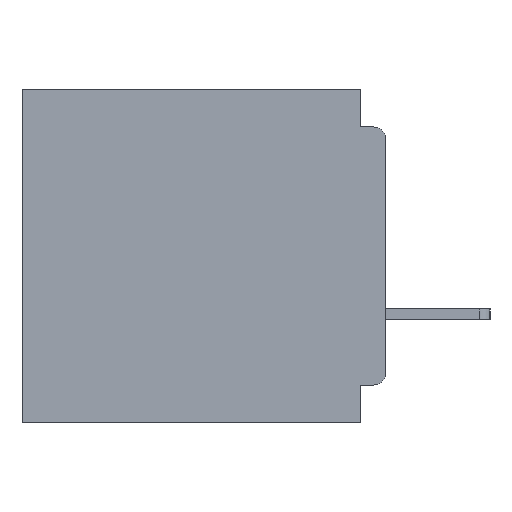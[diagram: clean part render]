
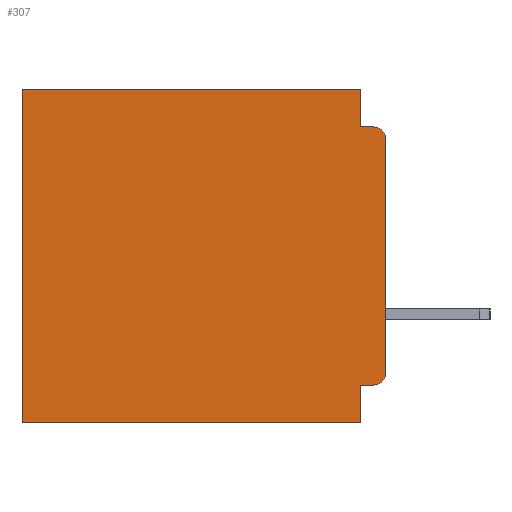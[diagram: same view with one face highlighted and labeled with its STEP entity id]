
A CAD part, left-side view. The second image highlights one B-rep face of the part: STEP entity #307.
In plain terms, the highlighted planar face has unit normal (-1, 0, 0).
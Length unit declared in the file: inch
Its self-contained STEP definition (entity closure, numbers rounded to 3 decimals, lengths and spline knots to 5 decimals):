
#307 = ADVANCED_FACE ( 'NONE', ( #13955 ), #12984, .F. ) ;
#2194 = VERTEX_POINT ( 'NONE', #8415 ) ;
#2566 = ORIENTED_EDGE ( 'NONE', *, *, #21219, .F. ) ;
#2774 = CIRCLE ( 'NONE', #42842, 0.015 ) ;
#2829 = EDGE_CURVE ( 'NONE', #35347, #46793, #45734, .T. ) ;
#4484 = DIRECTION ( 'NONE',  ( 0., 1., 0. ) ) ;
#4577 = DIRECTION ( 'NONE',  ( 0., 0., -1. ) ) ;
#4586 = EDGE_CURVE ( 'NONE', #9026, #2194, #24603, .T. ) ;
#5532 = VECTOR ( 'NONE', #4577, 39.37008 ) ;
#6021 = VECTOR ( 'NONE', #36018, 39.37008 ) ;
#7774 = DIRECTION ( 'NONE',  ( 0., 0., -1. ) ) ;
#8253 = VERTEX_POINT ( 'NONE', #26258 ) ;
#8362 = CARTESIAN_POINT ( 'NONE',  ( 0.3, 0., -0.355 ) ) ;
#8415 = CARTESIAN_POINT ( 'NONE',  ( 0.3, 0.031, -0.355 ) ) ;
#8632 = CARTESIAN_POINT ( 'NONE',  ( 0.3, 0.015, -0.06 ) ) ;
#8735 = EDGE_LOOP ( 'NONE', ( #28200, #45523, #2566, #38911, #15509, #45857, #46171, #40517, #16351, #39233 ) ) ;
#9026 = VERTEX_POINT ( 'NONE', #43619 ) ;
#10366 = CARTESIAN_POINT ( 'NONE',  ( 0.3, 0.031, 0. ) ) ;
#10535 = DIRECTION ( 'NONE',  ( 0., 0., -1. ) ) ;
#11523 = CARTESIAN_POINT ( 'NONE',  ( 0.3, 0., -0.06 ) ) ;
#11654 = DIRECTION ( 'NONE',  ( 1., 0., 0. ) ) ;
#11689 = LINE ( 'NONE', #12355, #31371 ) ;
#11791 = CARTESIAN_POINT ( 'NONE',  ( 0.3, 0.437, 0. ) ) ;
#11833 = DIRECTION ( 'NONE',  ( 0., 0., -1. ) ) ;
#12355 = CARTESIAN_POINT ( 'NONE',  ( 0.3, 0., 0. ) ) ;
#12660 = DIRECTION ( 'NONE',  ( 0., 0., -1. ) ) ;
#12862 = CARTESIAN_POINT ( 'NONE',  ( 0.3, 0., -0.4 ) ) ;
#12984 = PLANE ( 'NONE',  #39547 ) ;
#13205 = VERTEX_POINT ( 'NONE', #11791 ) ;
#13649 = EDGE_CURVE ( 'NONE', #39334, #19776, #18871, .T. ) ;
#13955 = FACE_OUTER_BOUND ( 'NONE', #8735, .T. ) ;
#15204 = EDGE_CURVE ( 'NONE', #2194, #35347, #24833, .T. ) ;
#15509 = ORIENTED_EDGE ( 'NONE', *, *, #23917, .T. ) ;
#15935 = DIRECTION ( 'NONE',  ( -1., 0., 0. ) ) ;
#16156 = LINE ( 'NONE', #20399, #5532 ) ;
#16351 = ORIENTED_EDGE ( 'NONE', *, *, #4586, .F. ) ;
#16360 = CARTESIAN_POINT ( 'NONE',  ( 0.3, 0., -0.4 ) ) ;
#16478 = VECTOR ( 'NONE', #10535, 39.37008 ) ;
#16972 = LINE ( 'NONE', #10366, #26156 ) ;
#18152 = LINE ( 'NONE', #47400, #48321 ) ;
#18871 = CIRCLE ( 'NONE', #40965, 0.015 ) ;
#19776 = VERTEX_POINT ( 'NONE', #46160 ) ;
#20399 = CARTESIAN_POINT ( 'NONE',  ( 0.3, 0., -0.4 ) ) ;
#21219 = EDGE_CURVE ( 'NONE', #8253, #19776, #18152, .T. ) ;
#21302 = CARTESIAN_POINT ( 'NONE',  ( 0.3, 0.031, -0.4 ) ) ;
#22746 = EDGE_CURVE ( 'NONE', #39334, #50909, #16156, .T. ) ;
#23603 = VECTOR ( 'NONE', #7774, 39.37008 ) ;
#23917 = EDGE_CURVE ( 'NONE', #28361, #13205, #11689, .T. ) ;
#24603 = LINE ( 'NONE', #8362, #6021 ) ;
#24789 = VECTOR ( 'NONE', #4484, 39.37008 ) ;
#24833 = LINE ( 'NONE', #51060, #23603 ) ;
#26156 = VECTOR ( 'NONE', #45822, 39.37008 ) ;
#26258 = CARTESIAN_POINT ( 'NONE',  ( 0.3, 0.031, -0.045 ) ) ;
#26896 = LINE ( 'NONE', #45812, #16478 ) ;
#27580 = EDGE_CURVE ( 'NONE', #13205, #46793, #26896, .T. ) ;
#27777 = DIRECTION ( 'NONE',  ( 0., -1., 0. ) ) ;
#28200 = ORIENTED_EDGE ( 'NONE', *, *, #22746, .F. ) ;
#28361 = VERTEX_POINT ( 'NONE', #39059 ) ;
#29354 = EDGE_CURVE ( 'NONE', #28361, #8253, #16972, .T. ) ;
#31371 = VECTOR ( 'NONE', #39918, 39.37008 ) ;
#35347 = VERTEX_POINT ( 'NONE', #21302 ) ;
#36018 = DIRECTION ( 'NONE',  ( 0., 1., 0. ) ) ;
#36281 = DIRECTION ( 'NONE',  ( -1., 0., 0. ) ) ;
#38911 = ORIENTED_EDGE ( 'NONE', *, *, #29354, .F. ) ;
#39059 = CARTESIAN_POINT ( 'NONE',  ( 0.3, 0.031, 0. ) ) ;
#39233 = ORIENTED_EDGE ( 'NONE', *, *, #49885, .T. ) ;
#39334 = VERTEX_POINT ( 'NONE', #11523 ) ;
#39516 = CARTESIAN_POINT ( 'NONE',  ( 0.3, 0.015, -0.34 ) ) ;
#39547 = AXIS2_PLACEMENT_3D ( 'NONE', #12862, #11654, #11833 ) ;
#39607 = CARTESIAN_POINT ( 'NONE',  ( 0.3, 0.437, -0.4 ) ) ;
#39918 = DIRECTION ( 'NONE',  ( 0., 1., 0. ) ) ;
#40517 = ORIENTED_EDGE ( 'NONE', *, *, #15204, .F. ) ;
#40965 = AXIS2_PLACEMENT_3D ( 'NONE', #8632, #36281, #12660 ) ;
#42472 = CARTESIAN_POINT ( 'NONE',  ( 0.3, 0., -0.34 ) ) ;
#42842 = AXIS2_PLACEMENT_3D ( 'NONE', #39516, #15935, #43440 ) ;
#43440 = DIRECTION ( 'NONE',  ( 0., 0., -1. ) ) ;
#43619 = CARTESIAN_POINT ( 'NONE',  ( 0.3, 0.015, -0.355 ) ) ;
#45523 = ORIENTED_EDGE ( 'NONE', *, *, #13649, .T. ) ;
#45734 = LINE ( 'NONE', #16360, #24789 ) ;
#45812 = CARTESIAN_POINT ( 'NONE',  ( 0.3, 0.437, -0.4 ) ) ;
#45822 = DIRECTION ( 'NONE',  ( 0., 0., -1. ) ) ;
#45857 = ORIENTED_EDGE ( 'NONE', *, *, #27580, .T. ) ;
#46160 = CARTESIAN_POINT ( 'NONE',  ( 0.3, 0.015, -0.045 ) ) ;
#46171 = ORIENTED_EDGE ( 'NONE', *, *, #2829, .F. ) ;
#46793 = VERTEX_POINT ( 'NONE', #39607 ) ;
#47400 = CARTESIAN_POINT ( 'NONE',  ( 0.3, 0., -0.045 ) ) ;
#48321 = VECTOR ( 'NONE', #27777, 39.37008 ) ;
#49885 = EDGE_CURVE ( 'NONE', #9026, #50909, #2774, .T. ) ;
#50909 = VERTEX_POINT ( 'NONE', #42472 ) ;
#51060 = CARTESIAN_POINT ( 'NONE',  ( 0.3, 0.031, -0.4 ) ) ;
